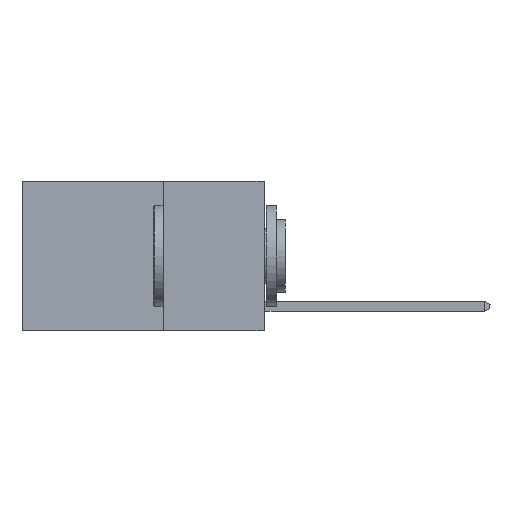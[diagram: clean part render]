
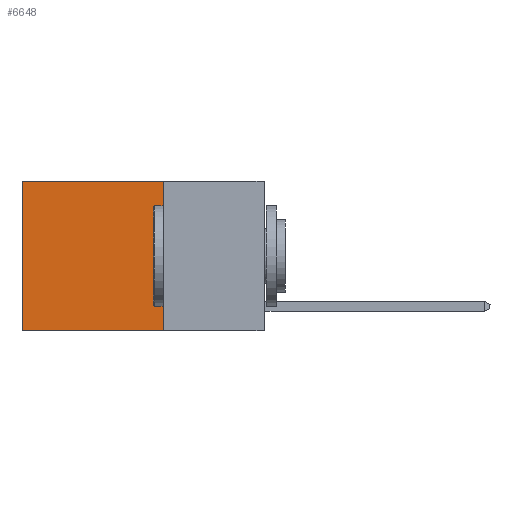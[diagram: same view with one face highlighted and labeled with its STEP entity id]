
A CAD part, left-side view. The second image highlights one B-rep face of the part: STEP entity #6648.
In plain terms, the highlighted planar face has unit normal (-1, 0, 0).
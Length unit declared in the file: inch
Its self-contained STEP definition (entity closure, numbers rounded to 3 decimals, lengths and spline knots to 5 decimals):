
#1022 = FACE_OUTER_BOUND ( 'NONE', #5089, .T. ) ;
#2147 = CARTESIAN_POINT ( 'NONE',  ( 0.2625, 0.6, 0. ) ) ;
#2469 = CARTESIAN_POINT ( 'NONE',  ( 0.2625, 0.25, 0. ) ) ;
#2816 = ORIENTED_EDGE ( 'NONE', *, *, #18119, .F. ) ;
#2904 = CARTESIAN_POINT ( 'NONE',  ( 0.2625, 0.25, 0. ) ) ;
#3264 = EDGE_CURVE ( 'NONE', #19384, #9325, #5131, .T. ) ;
#3469 = CARTESIAN_POINT ( 'NONE',  ( 0.2625, 0.25, -0.37 ) ) ;
#3830 = CARTESIAN_POINT ( 'NONE',  ( 0.2625, 0.25, 0. ) ) ;
#5089 = EDGE_LOOP ( 'NONE', ( #8026, #11808, #2816, #18265 ) ) ;
#5131 = LINE ( 'NONE', #2147, #14311 ) ;
#5512 = DIRECTION ( 'NONE',  ( 1., 0., 0. ) ) ;
#5879 = CARTESIAN_POINT ( 'NONE',  ( 0.2625, 0.6, 0. ) ) ;
#6359 = VECTOR ( 'NONE', #12745, 39.37008 ) ;
#6648 = ADVANCED_FACE ( 'NONE', ( #1022 ), #20121, .F. ) ;
#7340 = CARTESIAN_POINT ( 'NONE',  ( 0.2625, 0.6, -0.37 ) ) ;
#8026 = ORIENTED_EDGE ( 'NONE', *, *, #3264, .T. ) ;
#8509 = VECTOR ( 'NONE', #10050, 39.37008 ) ;
#8745 = DIRECTION ( 'NONE',  ( 0., 0., -1. ) ) ;
#9325 = VERTEX_POINT ( 'NONE', #7340 ) ;
#10050 = DIRECTION ( 'NONE',  ( 0., 1., 0. ) ) ;
#11487 = VECTOR ( 'NONE', #20540, 39.37008 ) ;
#11808 = ORIENTED_EDGE ( 'NONE', *, *, #20203, .F. ) ;
#12745 = DIRECTION ( 'NONE',  ( 0., 1., 0. ) ) ;
#12834 = LINE ( 'NONE', #3469, #8509 ) ;
#14115 = AXIS2_PLACEMENT_3D ( 'NONE', #3830, #5512, #16900 ) ;
#14220 = EDGE_CURVE ( 'NONE', #14791, #19384, #14985, .T. ) ;
#14311 = VECTOR ( 'NONE', #8745, 39.37008 ) ;
#14791 = VERTEX_POINT ( 'NONE', #21031 ) ;
#14985 = LINE ( 'NONE', #2904, #6359 ) ;
#16348 = LINE ( 'NONE', #2469, #11487 ) ;
#16900 = DIRECTION ( 'NONE',  ( 0., 0., -1. ) ) ;
#16928 = CARTESIAN_POINT ( 'NONE',  ( 0.2625, 0.25, -0.37 ) ) ;
#17095 = VERTEX_POINT ( 'NONE', #16928 ) ;
#18119 = EDGE_CURVE ( 'NONE', #14791, #17095, #16348, .T. ) ;
#18265 = ORIENTED_EDGE ( 'NONE', *, *, #14220, .T. ) ;
#19384 = VERTEX_POINT ( 'NONE', #5879 ) ;
#20121 = PLANE ( 'NONE',  #14115 ) ;
#20203 = EDGE_CURVE ( 'NONE', #17095, #9325, #12834, .T. ) ;
#20540 = DIRECTION ( 'NONE',  ( 0., 0., -1. ) ) ;
#21031 = CARTESIAN_POINT ( 'NONE',  ( 0.2625, 0.25, 0. ) ) ;
